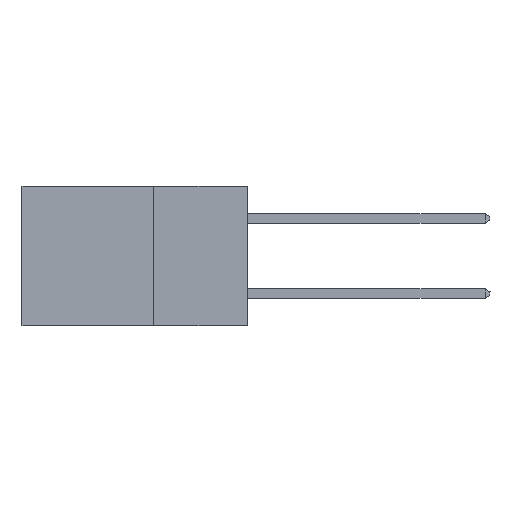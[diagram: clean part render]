
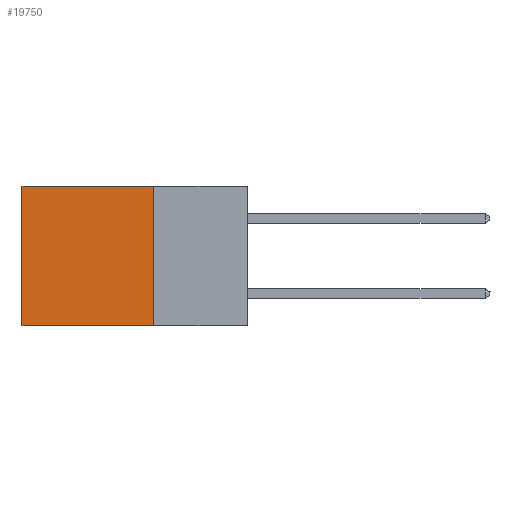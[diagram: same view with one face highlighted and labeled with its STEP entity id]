
A CAD part, left-side view. The second image highlights one B-rep face of the part: STEP entity #19750.
In plain terms, the highlighted planar face has unit normal (-1, 0, 0).
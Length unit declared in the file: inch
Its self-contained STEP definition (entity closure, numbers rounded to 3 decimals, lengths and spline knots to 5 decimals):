
#307 = DIRECTION ( 'NONE',  ( 0., 1., 0. ) ) ;
#2123 = CARTESIAN_POINT ( 'NONE',  ( 0.2615, 0.25, -0.37 ) ) ;
#3151 = CARTESIAN_POINT ( 'NONE',  ( 0.2615, 0.25, 0. ) ) ;
#3304 = DIRECTION ( 'NONE',  ( 0., 1., 0. ) ) ;
#3966 = ORIENTED_EDGE ( 'NONE', *, *, #7342, .T. ) ;
#4083 = DIRECTION ( 'NONE',  ( 0., 0., -1. ) ) ;
#4367 = LINE ( 'NONE', #10981, #13770 ) ;
#4526 = LINE ( 'NONE', #12723, #9555 ) ;
#5390 = CARTESIAN_POINT ( 'NONE',  ( 0.2615, 0.6, 0. ) ) ;
#6141 = LINE ( 'NONE', #23081, #10515 ) ;
#7342 = EDGE_CURVE ( 'NONE', #15905, #9385, #4367, .T. ) ;
#8163 = ORIENTED_EDGE ( 'NONE', *, *, #18188, .T. ) ;
#8814 = PLANE ( 'NONE',  #14719 ) ;
#8940 = ORIENTED_EDGE ( 'NONE', *, *, #22715, .F. ) ;
#9385 = VERTEX_POINT ( 'NONE', #13987 ) ;
#9555 = VECTOR ( 'NONE', #3304, 39.37008 ) ;
#9901 = VECTOR ( 'NONE', #4083, 39.37008 ) ;
#10135 = EDGE_CURVE ( 'NONE', #22815, #9385, #4526, .T. ) ;
#10515 = VECTOR ( 'NONE', #307, 39.37008 ) ;
#10683 = DIRECTION ( 'NONE',  ( 0., 0., -1. ) ) ;
#10729 = FACE_OUTER_BOUND ( 'NONE', #18642, .T. ) ;
#10981 = CARTESIAN_POINT ( 'NONE',  ( 0.2615, 0.6, -0.37 ) ) ;
#12723 = CARTESIAN_POINT ( 'NONE',  ( 0.2615, 0.25, -0.37 ) ) ;
#13770 = VECTOR ( 'NONE', #24259, 39.37008 ) ;
#13987 = CARTESIAN_POINT ( 'NONE',  ( 0.2615, 0.6, -0.37 ) ) ;
#14384 = CARTESIAN_POINT ( 'NONE',  ( 0.2615, 0.25, -0.37 ) ) ;
#14719 = AXIS2_PLACEMENT_3D ( 'NONE', #14384, #22033, #10683 ) ;
#15905 = VERTEX_POINT ( 'NONE', #5390 ) ;
#18188 = EDGE_CURVE ( 'NONE', #19230, #15905, #6141, .T. ) ;
#18642 = EDGE_LOOP ( 'NONE', ( #3966, #22615, #8940, #8163 ) ) ;
#19230 = VERTEX_POINT ( 'NONE', #3151 ) ;
#19750 = ADVANCED_FACE ( 'NONE', ( #10729 ), #8814, .F. ) ;
#20542 = LINE ( 'NONE', #2123, #9901 ) ;
#22033 = DIRECTION ( 'NONE',  ( 1., 0., 0. ) ) ;
#22615 = ORIENTED_EDGE ( 'NONE', *, *, #10135, .F. ) ;
#22715 = EDGE_CURVE ( 'NONE', #19230, #22815, #20542, .T. ) ;
#22815 = VERTEX_POINT ( 'NONE', #23183 ) ;
#23081 = CARTESIAN_POINT ( 'NONE',  ( 0.2615, 0.25, 0. ) ) ;
#23183 = CARTESIAN_POINT ( 'NONE',  ( 0.2615, 0.25, -0.37 ) ) ;
#24259 = DIRECTION ( 'NONE',  ( 0., 0., -1. ) ) ;
